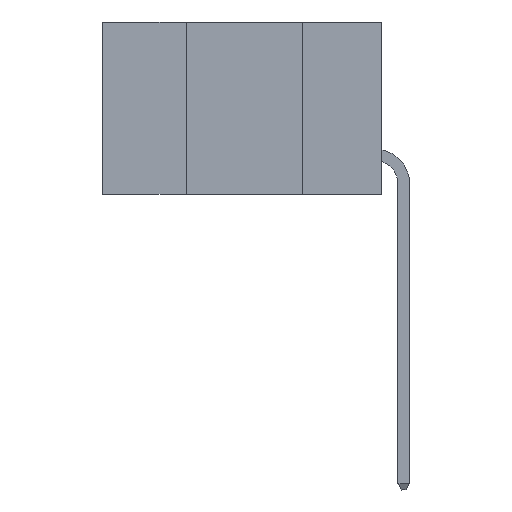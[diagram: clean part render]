
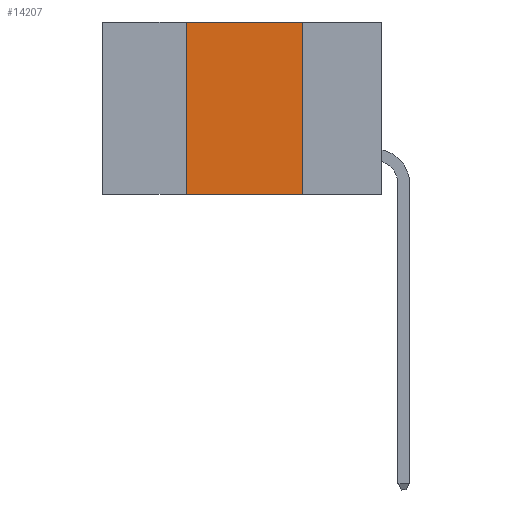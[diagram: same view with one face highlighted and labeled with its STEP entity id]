
A CAD part, left-side view. The second image highlights one B-rep face of the part: STEP entity #14207.
In plain terms, the highlighted planar face has unit normal (-1, 0, 0).
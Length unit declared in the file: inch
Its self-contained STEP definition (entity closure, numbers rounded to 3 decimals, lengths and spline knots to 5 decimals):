
#549 = CARTESIAN_POINT ( 'NONE',  ( 0., 0.17, 0. ) ) ;
#568 = VECTOR ( 'NONE', #6493, 39.37008 ) ;
#1135 = ORIENTED_EDGE ( 'NONE', *, *, #4617, .F. ) ;
#1228 = CARTESIAN_POINT ( 'NONE',  ( 0., 0.6, 0. ) ) ;
#1244 = ORIENTED_EDGE ( 'NONE', *, *, #8765, .T. ) ;
#1995 = AXIS2_PLACEMENT_3D ( 'NONE', #2644, #6104, #13868 ) ;
#2309 = LINE ( 'NONE', #1228, #10617 ) ;
#2644 = CARTESIAN_POINT ( 'NONE',  ( 0., 0.6, 0. ) ) ;
#3122 = FACE_OUTER_BOUND ( 'NONE', #10144, .T. ) ;
#3373 = LINE ( 'NONE', #13480, #6086 ) ;
#3973 = ORIENTED_EDGE ( 'NONE', *, *, #4528, .F. ) ;
#4125 = DIRECTION ( 'NONE',  ( 0., -1., 0. ) ) ;
#4528 = EDGE_CURVE ( 'NONE', #11817, #13436, #3373, .T. ) ;
#4617 = EDGE_CURVE ( 'NONE', #13436, #12739, #2309, .T. ) ;
#5698 = CARTESIAN_POINT ( 'NONE',  ( 0., 0.42, 0. ) ) ;
#6027 = VECTOR ( 'NONE', #12513, 39.37008 ) ;
#6086 = VECTOR ( 'NONE', #12961, 39.37008 ) ;
#6104 = DIRECTION ( 'NONE',  ( 1., 0., 0. ) ) ;
#6493 = DIRECTION ( 'NONE',  ( 0., -1., 0. ) ) ;
#8623 = LINE ( 'NONE', #11383, #6027 ) ;
#8765 = EDGE_CURVE ( 'NONE', #11817, #12087, #12269, .T. ) ;
#10144 = EDGE_LOOP ( 'NONE', ( #11053, #1135, #3973, #1244 ) ) ;
#10159 = CARTESIAN_POINT ( 'NONE',  ( 0., 0.42, -0.37 ) ) ;
#10597 = CARTESIAN_POINT ( 'NONE',  ( 0., 0.17, -0.37 ) ) ;
#10617 = VECTOR ( 'NONE', #4125, 39.37008 ) ;
#11053 = ORIENTED_EDGE ( 'NONE', *, *, #14049, .F. ) ;
#11383 = CARTESIAN_POINT ( 'NONE',  ( 0., 0.17, 0. ) ) ;
#11678 = PLANE ( 'NONE',  #1995 ) ;
#11817 = VERTEX_POINT ( 'NONE', #10159 ) ;
#12087 = VERTEX_POINT ( 'NONE', #10597 ) ;
#12269 = LINE ( 'NONE', #14228, #568 ) ;
#12513 = DIRECTION ( 'NONE',  ( 0., 0., -1. ) ) ;
#12739 = VERTEX_POINT ( 'NONE', #549 ) ;
#12961 = DIRECTION ( 'NONE',  ( 0., 0., 1. ) ) ;
#13436 = VERTEX_POINT ( 'NONE', #5698 ) ;
#13480 = CARTESIAN_POINT ( 'NONE',  ( 0., 0.42, 0. ) ) ;
#13868 = DIRECTION ( 'NONE',  ( 0., 0., -1. ) ) ;
#14049 = EDGE_CURVE ( 'NONE', #12739, #12087, #8623, .T. ) ;
#14207 = ADVANCED_FACE ( 'NONE', ( #3122 ), #11678, .F. ) ;
#14228 = CARTESIAN_POINT ( 'NONE',  ( 0., 0.6, -0.37 ) ) ;
